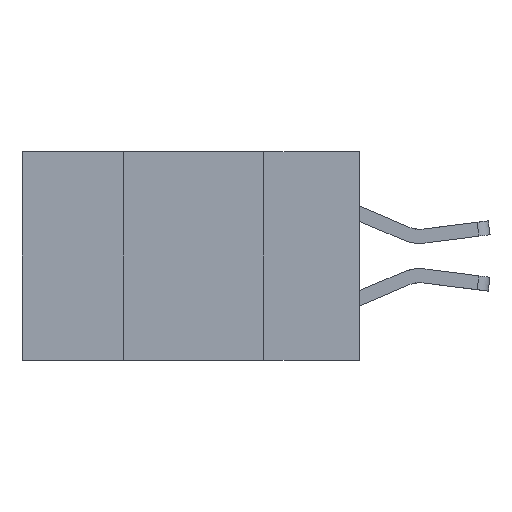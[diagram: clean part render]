
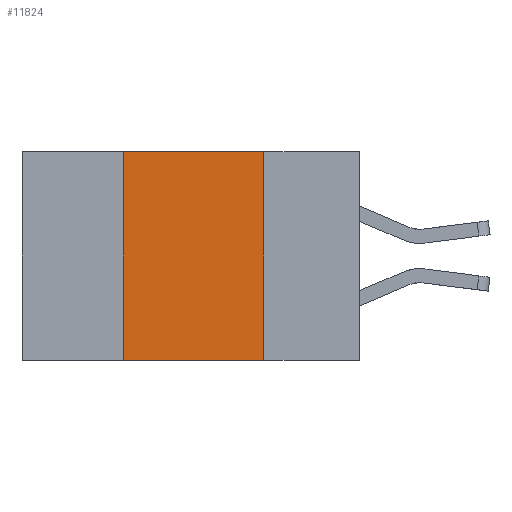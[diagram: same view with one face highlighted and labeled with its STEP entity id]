
A CAD part, left-side view. The second image highlights one B-rep face of the part: STEP entity #11824.
In plain terms, the highlighted planar face has unit normal (-1, 0, 0).
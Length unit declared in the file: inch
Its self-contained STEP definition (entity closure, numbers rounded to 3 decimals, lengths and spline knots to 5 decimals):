
#576 = DIRECTION ( 'NONE',  ( 0., -1., 0. ) ) ;
#799 = DIRECTION ( 'NONE',  ( 0., -1., 0. ) ) ;
#1425 = EDGE_CURVE ( 'NONE', #2108, #7369, #4861, .T. ) ;
#1479 = EDGE_CURVE ( 'NONE', #2108, #13082, #13367, .T. ) ;
#1514 = VECTOR ( 'NONE', #576, 39.37008 ) ;
#1530 = EDGE_CURVE ( 'NONE', #11885, #7369, #2515, .T. ) ;
#2108 = VERTEX_POINT ( 'NONE', #5078 ) ;
#2515 = LINE ( 'NONE', #10138, #14935 ) ;
#3181 = EDGE_CURVE ( 'NONE', #13082, #11885, #5969, .T. ) ;
#3199 = DIRECTION ( 'NONE',  ( 0., 0., 1. ) ) ;
#3295 = ORIENTED_EDGE ( 'NONE', *, *, #1425, .T. ) ;
#4861 = LINE ( 'NONE', #7656, #1514 ) ;
#5078 = CARTESIAN_POINT ( 'NONE',  ( 0., 0.42, -0.37 ) ) ;
#5418 = PLANE ( 'NONE',  #5542 ) ;
#5542 = AXIS2_PLACEMENT_3D ( 'NONE', #13838, #6701, #14949 ) ;
#5969 = LINE ( 'NONE', #14275, #8924 ) ;
#6701 = DIRECTION ( 'NONE',  ( 1., 0., 0. ) ) ;
#7028 = VECTOR ( 'NONE', #3199, 39.37008 ) ;
#7369 = VERTEX_POINT ( 'NONE', #10082 ) ;
#7656 = CARTESIAN_POINT ( 'NONE',  ( 0., 0.6, -0.37 ) ) ;
#8229 = EDGE_LOOP ( 'NONE', ( #12312, #15278, #15625, #3295 ) ) ;
#8924 = VECTOR ( 'NONE', #799, 39.37008 ) ;
#9016 = CARTESIAN_POINT ( 'NONE',  ( 0., 0.42, 0. ) ) ;
#10082 = CARTESIAN_POINT ( 'NONE',  ( 0., 0.17, -0.37 ) ) ;
#10138 = CARTESIAN_POINT ( 'NONE',  ( 0., 0.17, 0. ) ) ;
#10554 = CARTESIAN_POINT ( 'NONE',  ( 0., 0.42, 0. ) ) ;
#11824 = ADVANCED_FACE ( 'NONE', ( #14910 ), #5418, .F. ) ;
#11860 = DIRECTION ( 'NONE',  ( 0., 0., -1. ) ) ;
#11885 = VERTEX_POINT ( 'NONE', #15002 ) ;
#12312 = ORIENTED_EDGE ( 'NONE', *, *, #1530, .F. ) ;
#13082 = VERTEX_POINT ( 'NONE', #9016 ) ;
#13367 = LINE ( 'NONE', #10554, #7028 ) ;
#13838 = CARTESIAN_POINT ( 'NONE',  ( 0., 0.6, 0. ) ) ;
#14275 = CARTESIAN_POINT ( 'NONE',  ( 0., 0.6, 0. ) ) ;
#14910 = FACE_OUTER_BOUND ( 'NONE', #8229, .T. ) ;
#14935 = VECTOR ( 'NONE', #11860, 39.37008 ) ;
#14949 = DIRECTION ( 'NONE',  ( 0., 0., -1. ) ) ;
#15002 = CARTESIAN_POINT ( 'NONE',  ( 0., 0.17, 0. ) ) ;
#15278 = ORIENTED_EDGE ( 'NONE', *, *, #3181, .F. ) ;
#15625 = ORIENTED_EDGE ( 'NONE', *, *, #1479, .F. ) ;
